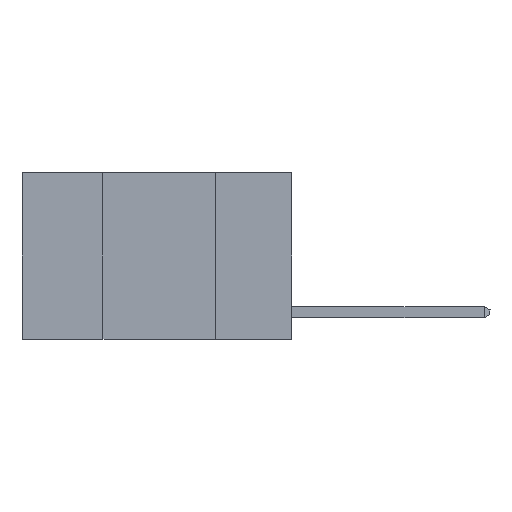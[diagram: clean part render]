
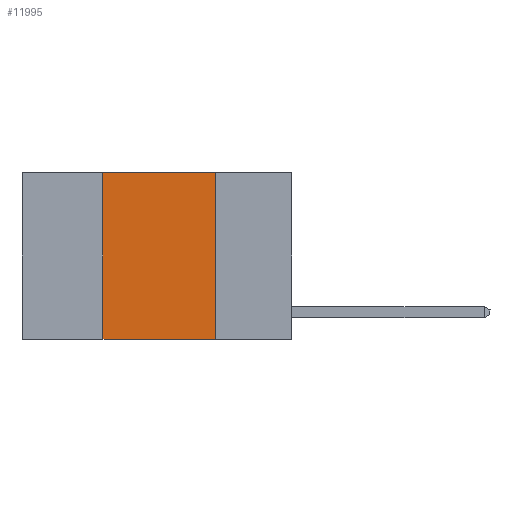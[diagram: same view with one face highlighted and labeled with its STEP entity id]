
A CAD part, left-side view. The second image highlights one B-rep face of the part: STEP entity #11995.
In plain terms, the highlighted planar face has unit normal (-1, 0, 0).
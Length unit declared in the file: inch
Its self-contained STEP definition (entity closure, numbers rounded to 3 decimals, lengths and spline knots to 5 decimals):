
#121 = LINE ( 'NONE', #12522, #13211 ) ;
#387 = DIRECTION ( 'NONE',  ( 0., 0., -1. ) ) ;
#1056 = LINE ( 'NONE', #4723, #18119 ) ;
#2511 = CARTESIAN_POINT ( 'NONE',  ( 0., 0.6, 0. ) ) ;
#2527 = EDGE_CURVE ( 'NONE', #19703, #21847, #10072, .T. ) ;
#4267 = DIRECTION ( 'NONE',  ( 0., 0., -1. ) ) ;
#4723 = CARTESIAN_POINT ( 'NONE',  ( 0., 0.6, 0. ) ) ;
#5371 = ORIENTED_EDGE ( 'NONE', *, *, #21193, .T. ) ;
#5550 = ORIENTED_EDGE ( 'NONE', *, *, #15229, .F. ) ;
#6442 = DIRECTION ( 'NONE',  ( 0., -1., 0. ) ) ;
#6649 = VERTEX_POINT ( 'NONE', #12998 ) ;
#9101 = DIRECTION ( 'NONE',  ( 0., -1., 0. ) ) ;
#9307 = AXIS2_PLACEMENT_3D ( 'NONE', #2511, #14438, #4267 ) ;
#9330 = PLANE ( 'NONE',  #9307 ) ;
#10072 = LINE ( 'NONE', #15304, #14024 ) ;
#10874 = CARTESIAN_POINT ( 'NONE',  ( 0., 0.42, 0. ) ) ;
#11995 = ADVANCED_FACE ( 'NONE', ( #17237 ), #9330, .F. ) ;
#12121 = VERTEX_POINT ( 'NONE', #18151 ) ;
#12357 = CARTESIAN_POINT ( 'NONE',  ( 0., 0.17, 0. ) ) ;
#12522 = CARTESIAN_POINT ( 'NONE',  ( 0., 0.6, -0.37 ) ) ;
#12998 = CARTESIAN_POINT ( 'NONE',  ( 0., 0.17, 0. ) ) ;
#13211 = VECTOR ( 'NONE', #9101, 39.37008 ) ;
#14024 = VECTOR ( 'NONE', #20408, 39.37008 ) ;
#14324 = ORIENTED_EDGE ( 'NONE', *, *, #18092, .F. ) ;
#14438 = DIRECTION ( 'NONE',  ( 1., 0., 0. ) ) ;
#15229 = EDGE_CURVE ( 'NONE', #21847, #6649, #1056, .T. ) ;
#15304 = CARTESIAN_POINT ( 'NONE',  ( 0., 0.42, 0. ) ) ;
#16243 = LINE ( 'NONE', #12357, #20198 ) ;
#17237 = FACE_OUTER_BOUND ( 'NONE', #18741, .T. ) ;
#18092 = EDGE_CURVE ( 'NONE', #6649, #12121, #16243, .T. ) ;
#18119 = VECTOR ( 'NONE', #6442, 39.37008 ) ;
#18151 = CARTESIAN_POINT ( 'NONE',  ( 0., 0.17, -0.37 ) ) ;
#18568 = CARTESIAN_POINT ( 'NONE',  ( 0., 0.42, -0.37 ) ) ;
#18741 = EDGE_LOOP ( 'NONE', ( #14324, #5550, #18934, #5371 ) ) ;
#18934 = ORIENTED_EDGE ( 'NONE', *, *, #2527, .F. ) ;
#19703 = VERTEX_POINT ( 'NONE', #18568 ) ;
#20198 = VECTOR ( 'NONE', #387, 39.37008 ) ;
#20408 = DIRECTION ( 'NONE',  ( 0., 0., 1. ) ) ;
#21193 = EDGE_CURVE ( 'NONE', #19703, #12121, #121, .T. ) ;
#21847 = VERTEX_POINT ( 'NONE', #10874 ) ;
